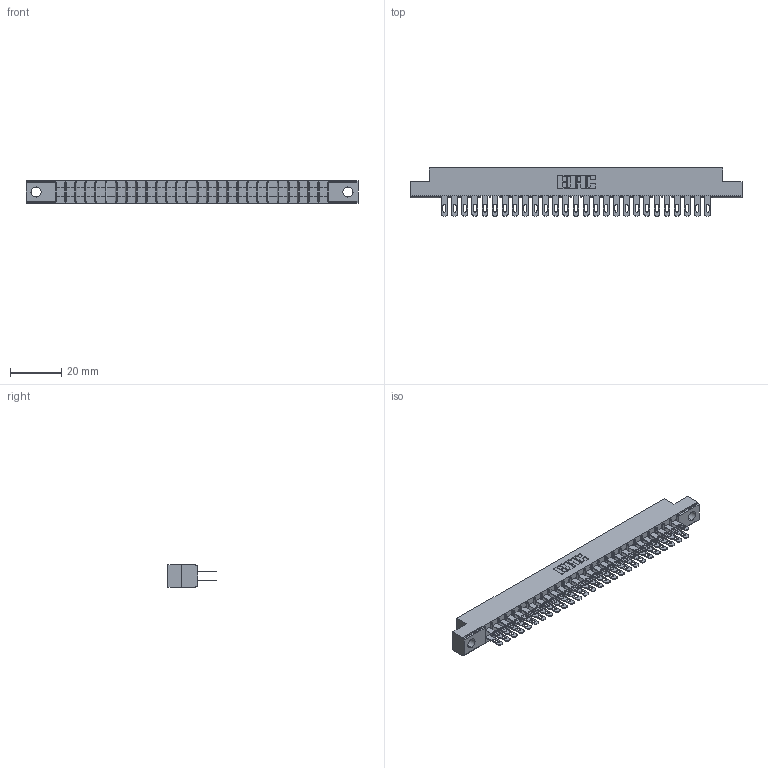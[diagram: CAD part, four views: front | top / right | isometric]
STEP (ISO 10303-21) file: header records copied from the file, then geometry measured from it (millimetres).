
FILE_DESCRIPTION (( 'STEP AP203' ), '1' );
FILE_NAME ('355-054-500-504.STEP', '2019-09-11T16:51:57', ( '' ), ( '' ), 'SwSTEP 2.0', 'SolidWorks 2016', '' );
FILE_SCHEMA (( 'CONFIG_CONTROL_DESIGN' ));
Length unit declared in the file: inch
Products named in the file (3): 355-054-500-504; 305 Part_.156 Dia; 305-290-001_500
Assembly tree (55 placements, depth 2):
  355-054-500-504
    305 Part_.156 Dia
    305-290-001_500  x54
Bounding box: 130 x 18.85 x 8.71 mm (x, y, z)
Volume: 7831.1 mm3; surface area: 16770 mm2
Topology: 55 solids, 55 shells, 2830 faces, 8101 edges, 5254 vertices
Faces by surface type: plane 1594, cylinder 1128, sphere 108
Entity records: 31500 total; most frequent: CARTESIAN_POINT 5217, ORIENTED_EDGE 5174, DIRECTION 5053, EDGE_CURVE 2587, VECTOR 2081, LINE 2081, VERTEX_POINT 1650, AXIS2_PLACEMENT_3D 1486
